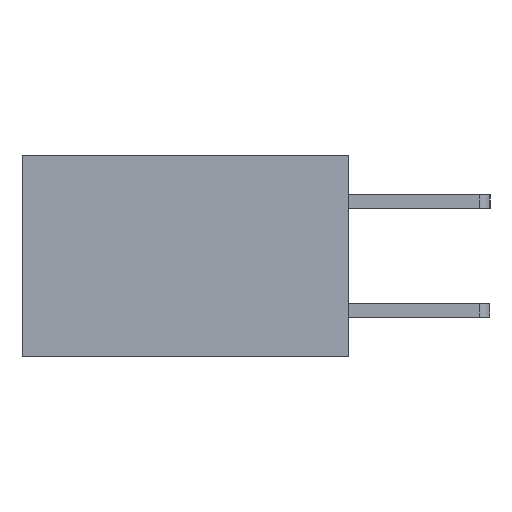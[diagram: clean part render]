
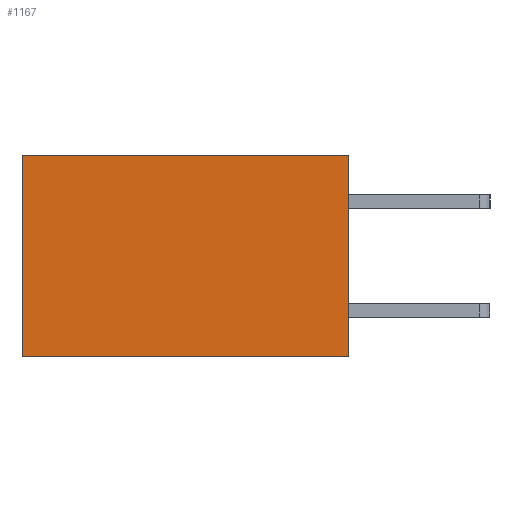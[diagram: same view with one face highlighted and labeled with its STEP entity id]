
A CAD part, left-side view. The second image highlights one B-rep face of the part: STEP entity #1167.
In plain terms, the highlighted planar face has unit normal (-1, 0, 0).
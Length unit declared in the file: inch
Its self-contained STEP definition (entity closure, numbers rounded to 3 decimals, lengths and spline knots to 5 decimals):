
#147 = EDGE_LOOP ( 'NONE', ( #2242, #2802, #3278, #5221 ) ) ;
#165 = VERTEX_POINT ( 'NONE', #3964 ) ;
#206 = CARTESIAN_POINT ( 'NONE',  ( 0.298, 0.6, -0.37 ) ) ;
#275 = DIRECTION ( 'NONE',  ( 0., 0., -1. ) ) ;
#525 = LINE ( 'NONE', #2056, #9859 ) ;
#587 = VERTEX_POINT ( 'NONE', #2769 ) ;
#627 = DIRECTION ( 'NONE',  ( 0., 1., 0. ) ) ;
#765 = AXIS2_PLACEMENT_3D ( 'NONE', #8830, #8633, #4411 ) ;
#1167 = ADVANCED_FACE ( 'NONE', ( #6485 ), #10349, .F. ) ;
#1527 = VECTOR ( 'NONE', #7571, 39.37008 ) ;
#1706 = CARTESIAN_POINT ( 'NONE',  ( 0.298, 0., 0. ) ) ;
#2056 = CARTESIAN_POINT ( 'NONE',  ( 0.298, 0., 0. ) ) ;
#2242 = ORIENTED_EDGE ( 'NONE', *, *, #3954, .T. ) ;
#2769 = CARTESIAN_POINT ( 'NONE',  ( 0.298, 0., -0.37 ) ) ;
#2802 = ORIENTED_EDGE ( 'NONE', *, *, #11117, .F. ) ;
#2917 = LINE ( 'NONE', #10057, #7717 ) ;
#3278 = ORIENTED_EDGE ( 'NONE', *, *, #10703, .F. ) ;
#3954 = EDGE_CURVE ( 'NONE', #165, #11183, #4206, .T. ) ;
#3964 = CARTESIAN_POINT ( 'NONE',  ( 0.298, 0.6, 0. ) ) ;
#4206 = LINE ( 'NONE', #9423, #1527 ) ;
#4411 = DIRECTION ( 'NONE',  ( 0., 0., -1. ) ) ;
#5221 = ORIENTED_EDGE ( 'NONE', *, *, #5516, .T. ) ;
#5516 = EDGE_CURVE ( 'NONE', #7118, #165, #10605, .T. ) ;
#5792 = CARTESIAN_POINT ( 'NONE',  ( 0.298, 0., 0. ) ) ;
#6485 = FACE_OUTER_BOUND ( 'NONE', #147, .T. ) ;
#7118 = VERTEX_POINT ( 'NONE', #1706 ) ;
#7571 = DIRECTION ( 'NONE',  ( 0., 0., -1. ) ) ;
#7717 = VECTOR ( 'NONE', #10900, 39.37008 ) ;
#8242 = VECTOR ( 'NONE', #627, 39.37008 ) ;
#8633 = DIRECTION ( 'NONE',  ( 1., 0., 0. ) ) ;
#8830 = CARTESIAN_POINT ( 'NONE',  ( 0.298, 0., 0. ) ) ;
#9423 = CARTESIAN_POINT ( 'NONE',  ( 0.298, 0.6, 0. ) ) ;
#9859 = VECTOR ( 'NONE', #275, 39.37008 ) ;
#10057 = CARTESIAN_POINT ( 'NONE',  ( 0.298, 0., -0.37 ) ) ;
#10349 = PLANE ( 'NONE',  #765 ) ;
#10605 = LINE ( 'NONE', #5792, #8242 ) ;
#10703 = EDGE_CURVE ( 'NONE', #7118, #587, #525, .T. ) ;
#10900 = DIRECTION ( 'NONE',  ( 0., 1., 0. ) ) ;
#11117 = EDGE_CURVE ( 'NONE', #587, #11183, #2917, .T. ) ;
#11183 = VERTEX_POINT ( 'NONE', #206 ) ;
